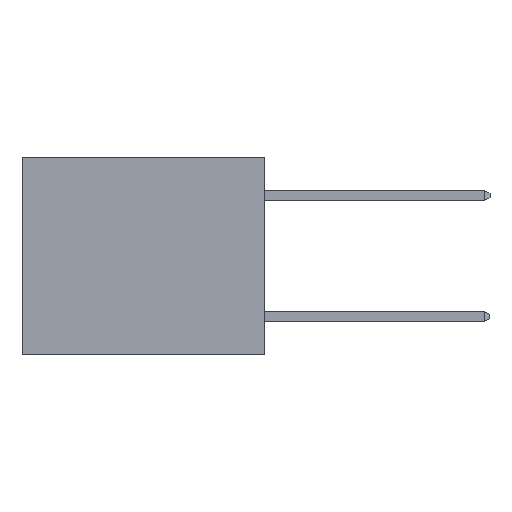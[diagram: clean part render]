
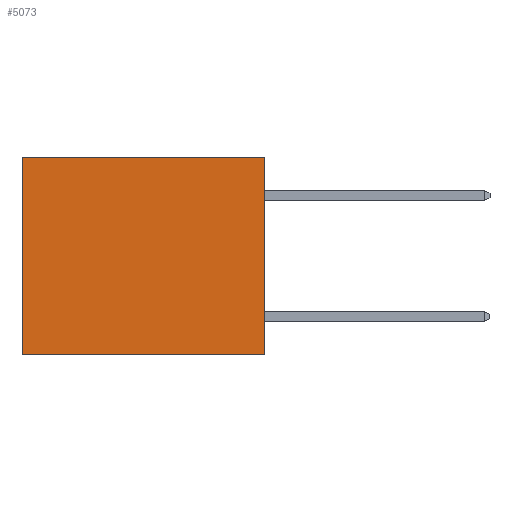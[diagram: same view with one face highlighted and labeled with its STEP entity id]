
A CAD part, left-side view. The second image highlights one B-rep face of the part: STEP entity #5073.
In plain terms, the highlighted planar face has unit normal (-1, 0, 0).
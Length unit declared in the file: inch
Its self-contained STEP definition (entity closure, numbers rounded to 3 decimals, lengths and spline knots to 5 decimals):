
#176 = EDGE_CURVE ( 'NONE', #7273, #4946, #8596, .T. ) ;
#358 = CARTESIAN_POINT ( 'NONE',  ( 0.3165, 0., 0. ) ) ;
#1035 = ORIENTED_EDGE ( 'NONE', *, *, #176, .F. ) ;
#1070 = AXIS2_PLACEMENT_3D ( 'NONE', #4981, #3493, #8264 ) ;
#1107 = LINE ( 'NONE', #1463, #8119 ) ;
#1156 = CARTESIAN_POINT ( 'NONE',  ( 0.3165, 0., -0.49 ) ) ;
#1402 = DIRECTION ( 'NONE',  ( 0., 0., -1. ) ) ;
#1406 = LINE ( 'NONE', #358, #2482 ) ;
#1463 = CARTESIAN_POINT ( 'NONE',  ( 0.3165, 0.6, -0.49 ) ) ;
#1511 = CARTESIAN_POINT ( 'NONE',  ( 0.3165, 0., 0. ) ) ;
#2073 = ORIENTED_EDGE ( 'NONE', *, *, #2467, .F. ) ;
#2242 = EDGE_CURVE ( 'NONE', #6376, #4946, #1107, .T. ) ;
#2467 = EDGE_CURVE ( 'NONE', #2651, #7273, #5992, .T. ) ;
#2482 = VECTOR ( 'NONE', #3159, 39.37008 ) ;
#2508 = EDGE_LOOP ( 'NONE', ( #4196, #1035, #2073, #8670 ) ) ;
#2651 = VERTEX_POINT ( 'NONE', #1511 ) ;
#3159 = DIRECTION ( 'NONE',  ( 0., 1., 0. ) ) ;
#3493 = DIRECTION ( 'NONE',  ( 1., 0., 0. ) ) ;
#3544 = VECTOR ( 'NONE', #6469, 39.37008 ) ;
#4135 = EDGE_CURVE ( 'NONE', #2651, #6376, #1406, .T. ) ;
#4196 = ORIENTED_EDGE ( 'NONE', *, *, #2242, .T. ) ;
#4414 = CARTESIAN_POINT ( 'NONE',  ( 0.3165, 0., -0.49 ) ) ;
#4593 = DIRECTION ( 'NONE',  ( 0., 1., 0. ) ) ;
#4946 = VERTEX_POINT ( 'NONE', #5370 ) ;
#4981 = CARTESIAN_POINT ( 'NONE',  ( 0.3165, 0., -0.49 ) ) ;
#4986 = CARTESIAN_POINT ( 'NONE',  ( 0.3165, 0.6, 0. ) ) ;
#5073 = ADVANCED_FACE ( 'NONE', ( #7884 ), #7648, .F. ) ;
#5370 = CARTESIAN_POINT ( 'NONE',  ( 0.3165, 0.6, -0.49 ) ) ;
#5992 = LINE ( 'NONE', #4414, #3544 ) ;
#6376 = VERTEX_POINT ( 'NONE', #4986 ) ;
#6469 = DIRECTION ( 'NONE',  ( 0., 0., -1. ) ) ;
#6808 = VECTOR ( 'NONE', #4593, 39.37008 ) ;
#7273 = VERTEX_POINT ( 'NONE', #7280 ) ;
#7280 = CARTESIAN_POINT ( 'NONE',  ( 0.3165, 0., -0.49 ) ) ;
#7648 = PLANE ( 'NONE',  #1070 ) ;
#7884 = FACE_OUTER_BOUND ( 'NONE', #2508, .T. ) ;
#8119 = VECTOR ( 'NONE', #1402, 39.37008 ) ;
#8264 = DIRECTION ( 'NONE',  ( 0., 0., -1. ) ) ;
#8596 = LINE ( 'NONE', #1156, #6808 ) ;
#8670 = ORIENTED_EDGE ( 'NONE', *, *, #4135, .T. ) ;
